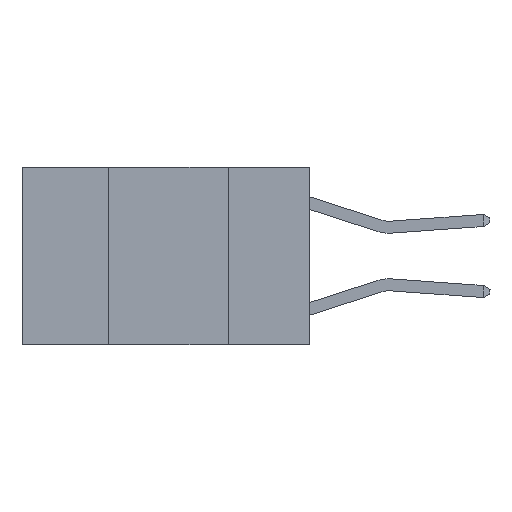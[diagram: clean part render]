
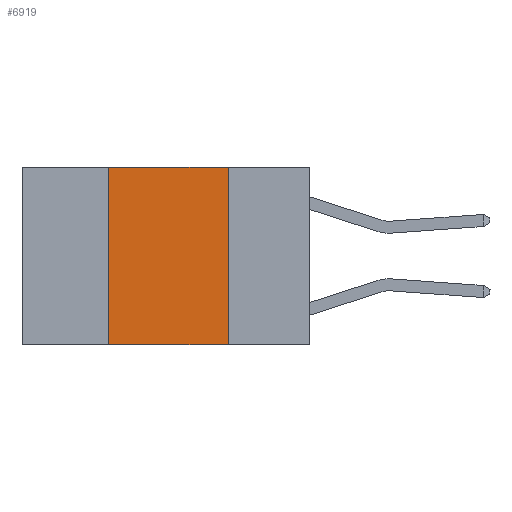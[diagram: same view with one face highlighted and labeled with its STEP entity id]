
A CAD part, left-side view. The second image highlights one B-rep face of the part: STEP entity #6919.
In plain terms, the highlighted planar face has unit normal (-1, 0, 0).
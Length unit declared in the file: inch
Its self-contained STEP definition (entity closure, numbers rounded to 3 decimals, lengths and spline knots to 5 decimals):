
#580 = DIRECTION ( 'NONE',  ( 0., -1., 0. ) ) ;
#604 = FACE_OUTER_BOUND ( 'NONE', #7832, .T. ) ;
#955 = LINE ( 'NONE', #1022, #7144 ) ;
#1022 = CARTESIAN_POINT ( 'NONE',  ( 0., 0.17, 0. ) ) ;
#1108 = ORIENTED_EDGE ( 'NONE', *, *, #9860, .F. ) ;
#1612 = AXIS2_PLACEMENT_3D ( 'NONE', #1805, #2664, #8424 ) ;
#1638 = CARTESIAN_POINT ( 'NONE',  ( 0., 0.42, 0. ) ) ;
#1775 = VERTEX_POINT ( 'NONE', #9906 ) ;
#1805 = CARTESIAN_POINT ( 'NONE',  ( 0., 0.6, 0. ) ) ;
#1919 = DIRECTION ( 'NONE',  ( 0., -1., 0. ) ) ;
#1933 = DIRECTION ( 'NONE',  ( 0., 0., -1. ) ) ;
#2500 = DIRECTION ( 'NONE',  ( 0., 0., 1. ) ) ;
#2664 = DIRECTION ( 'NONE',  ( 1., 0., 0. ) ) ;
#2800 = CARTESIAN_POINT ( 'NONE',  ( 0., 0.17, -0.37 ) ) ;
#2932 = ORIENTED_EDGE ( 'NONE', *, *, #8408, .T. ) ;
#3180 = VECTOR ( 'NONE', #2500, 39.37008 ) ;
#3231 = VERTEX_POINT ( 'NONE', #6161 ) ;
#3264 = VECTOR ( 'NONE', #1919, 39.37008 ) ;
#5139 = EDGE_CURVE ( 'NONE', #3231, #9567, #5740, .T. ) ;
#5150 = VECTOR ( 'NONE', #580, 39.37008 ) ;
#5585 = ORIENTED_EDGE ( 'NONE', *, *, #5139, .F. ) ;
#5740 = LINE ( 'NONE', #6120, #3264 ) ;
#6081 = ORIENTED_EDGE ( 'NONE', *, *, #9616, .F. ) ;
#6120 = CARTESIAN_POINT ( 'NONE',  ( 0., 0.6, 0. ) ) ;
#6161 = CARTESIAN_POINT ( 'NONE',  ( 0., 0.42, 0. ) ) ;
#6510 = CARTESIAN_POINT ( 'NONE',  ( 0., 0.6, -0.37 ) ) ;
#6772 = PLANE ( 'NONE',  #1612 ) ;
#6919 = ADVANCED_FACE ( 'NONE', ( #604 ), #6772, .F. ) ;
#7144 = VECTOR ( 'NONE', #1933, 39.37008 ) ;
#7380 = CARTESIAN_POINT ( 'NONE',  ( 0., 0.17, 0. ) ) ;
#7832 = EDGE_LOOP ( 'NONE', ( #1108, #5585, #6081, #2932 ) ) ;
#8408 = EDGE_CURVE ( 'NONE', #1775, #9871, #9472, .T. ) ;
#8424 = DIRECTION ( 'NONE',  ( 0., 0., -1. ) ) ;
#9472 = LINE ( 'NONE', #6510, #5150 ) ;
#9567 = VERTEX_POINT ( 'NONE', #7380 ) ;
#9616 = EDGE_CURVE ( 'NONE', #1775, #3231, #9945, .T. ) ;
#9860 = EDGE_CURVE ( 'NONE', #9567, #9871, #955, .T. ) ;
#9871 = VERTEX_POINT ( 'NONE', #2800 ) ;
#9906 = CARTESIAN_POINT ( 'NONE',  ( 0., 0.42, -0.37 ) ) ;
#9945 = LINE ( 'NONE', #1638, #3180 ) ;
